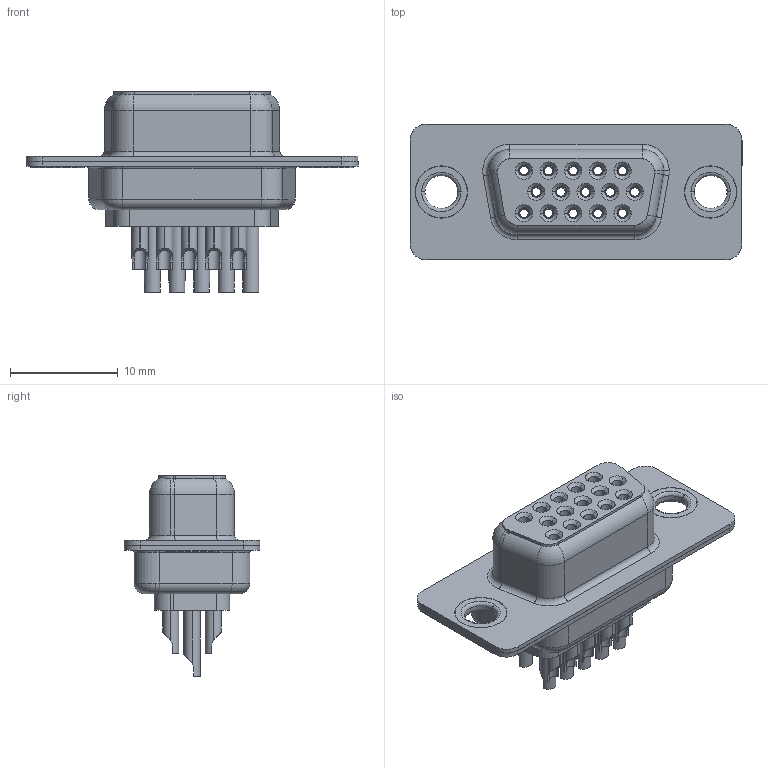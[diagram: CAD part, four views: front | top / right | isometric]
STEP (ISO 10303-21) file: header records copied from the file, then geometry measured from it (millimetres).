
FILE_DESCRIPTION (( 'STEP AP203' ), '1' );
FILE_NAME ('638-015-332-041.STEP', '2019-05-14T18:57:48', ( '' ), ( '' ), 'SwSTEP 2.0', 'SolidWorks 2016', '' );
FILE_SCHEMA (( 'CONFIG_CONTROL_DESIGN' ));
Length unit declared in the file: millimetre
Products named in the file (8): 638 Shell Front_15 Contacts; 638 Shell Rear_15 Contacts; 638 Contact Row 1_32L; 638 Contact Row 2_32L; 638 Contact Row 3_32L; 638 Thru Hole Rivet; 638-015-332-041; 638 Housing_15 Contacts
Assembly tree (20 placements, depth 2):
  638-015-332-041
    638 Housing_15 Contacts
    638 Shell Front_15 Contacts
    638 Shell Rear_15 Contacts
    638 Contact Row 1_32L  x5
    638 Contact Row 2_32L  x5
    638 Contact Row 3_32L  x5
    638 Thru Hole Rivet  x2
Bounding box: 30.81 x 12.6 x 18.6 mm (x, y, z)
Volume: 1524.8 mm3; surface area: 5714.5 mm2
Topology: 20 solids, 20 shells, 1588 faces, 3993 edges, 2501 vertices
Faces by surface type: cylinder 496, plane 382, torus 335, bspline 300, cone 75
Entity records: 22757 total; most frequent: CARTESIAN_POINT 6299, DIRECTION 3290, ORIENTED_EDGE 3154, EDGE_CURVE 1577, AXIS2_PLACEMENT_3D 1370, VERTEX_POINT 989, EDGE_LOOP 754, CIRCLE 751
